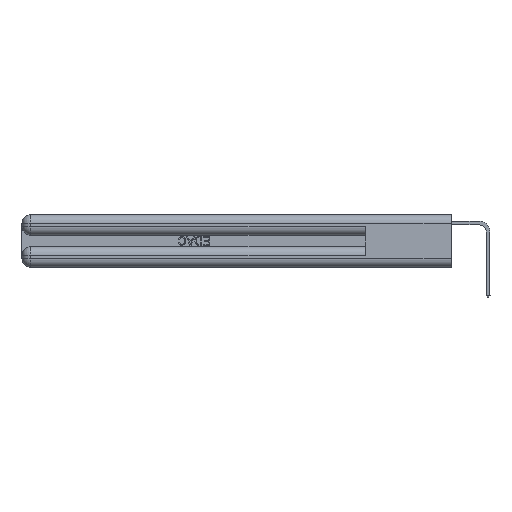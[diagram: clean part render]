
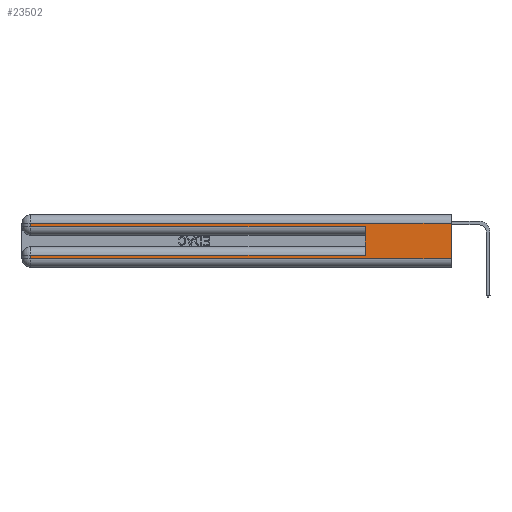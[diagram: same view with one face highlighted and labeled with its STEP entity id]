
A CAD part, left-side view. The second image highlights one B-rep face of the part: STEP entity #23502.
In plain terms, the highlighted planar face has unit normal (-1, 0, 0).
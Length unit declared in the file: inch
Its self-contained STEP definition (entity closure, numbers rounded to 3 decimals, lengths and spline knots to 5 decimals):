
#76 = VECTOR ( 'NONE', #25563, 39.37008 ) ;
#184 = CARTESIAN_POINT ( 'NONE',  ( 0., 2.94, 0.37 ) ) ;
#191 = VERTEX_POINT ( 'NONE', #11091 ) ;
#522 = CARTESIAN_POINT ( 'NONE',  ( 0., 0., 0.37 ) ) ;
#659 = ORIENTED_EDGE ( 'NONE', *, *, #31729, .T. ) ;
#1191 = CARTESIAN_POINT ( 'NONE',  ( 0., 2.94, 0.285 ) ) ;
#1357 = CARTESIAN_POINT ( 'NONE',  ( 0., 0.6, 0.285 ) ) ;
#1620 = ORIENTED_EDGE ( 'NONE', *, *, #3179, .T. ) ;
#1854 = ORIENTED_EDGE ( 'NONE', *, *, #27636, .F. ) ;
#2759 = LINE ( 'NONE', #522, #27994 ) ;
#3179 = EDGE_CURVE ( 'NONE', #11725, #24315, #15937, .T. ) ;
#3372 = VERTEX_POINT ( 'NONE', #1191 ) ;
#3619 = CARTESIAN_POINT ( 'NONE',  ( 0., 2.94, 0.085 ) ) ;
#3758 = EDGE_CURVE ( 'NONE', #26322, #11779, #14314, .T. ) ;
#4474 = EDGE_CURVE ( 'NONE', #24315, #31148, #29423, .T. ) ;
#5207 = EDGE_CURVE ( 'NONE', #33127, #3372, #30733, .T. ) ;
#6445 = VECTOR ( 'NONE', #21344, 39.37008 ) ;
#6697 = VECTOR ( 'NONE', #28147, 39.37008 ) ;
#7281 = DIRECTION ( 'NONE',  ( 1., 0., 0. ) ) ;
#8001 = ORIENTED_EDGE ( 'NONE', *, *, #3758, .F. ) ;
#8358 = VECTOR ( 'NONE', #28224, 39.37008 ) ;
#8670 = DIRECTION ( 'NONE',  ( 0., -1., 0. ) ) ;
#9128 = CARTESIAN_POINT ( 'NONE',  ( 0., 0.6, 0.145 ) ) ;
#9309 = EDGE_CURVE ( 'NONE', #3372, #11779, #12222, .T. ) ;
#9751 = ORIENTED_EDGE ( 'NONE', *, *, #4474, .T. ) ;
#11083 = CARTESIAN_POINT ( 'NONE',  ( 0., 0.6, 0.085 ) ) ;
#11091 = CARTESIAN_POINT ( 'NONE',  ( 0., 0., 0.31 ) ) ;
#11560 = CARTESIAN_POINT ( 'NONE',  ( 0., 2.94, 0.06 ) ) ;
#11604 = CARTESIAN_POINT ( 'NONE',  ( 0., 0., 0.06 ) ) ;
#11725 = VERTEX_POINT ( 'NONE', #3619 ) ;
#11779 = VERTEX_POINT ( 'NONE', #1357 ) ;
#11814 = CARTESIAN_POINT ( 'NONE',  ( 0., 0., 0.31 ) ) ;
#12222 = LINE ( 'NONE', #33140, #21683 ) ;
#12746 = CARTESIAN_POINT ( 'NONE',  ( 0., 0., 0.06 ) ) ;
#13017 = CARTESIAN_POINT ( 'NONE',  ( 0., 0., 0.37 ) ) ;
#13352 = DIRECTION ( 'NONE',  ( 0., 0., -1. ) ) ;
#14314 = LINE ( 'NONE', #9128, #6697 ) ;
#15551 = VECTOR ( 'NONE', #8670, 39.37008 ) ;
#15937 = LINE ( 'NONE', #184, #6445 ) ;
#17080 = DIRECTION ( 'NONE',  ( 0., -1., 0. ) ) ;
#17611 = CARTESIAN_POINT ( 'NONE',  ( 0., 2.94, 0.37 ) ) ;
#19448 = ORIENTED_EDGE ( 'NONE', *, *, #21286, .T. ) ;
#20329 = EDGE_LOOP ( 'NONE', ( #1854, #659, #26509, #27151, #8001, #19448, #1620, #9751 ) ) ;
#21286 = EDGE_CURVE ( 'NONE', #26322, #11725, #23200, .T. ) ;
#21344 = DIRECTION ( 'NONE',  ( 0., 0., -1. ) ) ;
#21683 = VECTOR ( 'NONE', #17080, 39.37008 ) ;
#23200 = LINE ( 'NONE', #33733, #31613 ) ;
#23502 = ADVANCED_FACE ( 'NONE', ( #28411 ), #31165, .F. ) ;
#23600 = DIRECTION ( 'NONE',  ( 0., 0., -1. ) ) ;
#24315 = VERTEX_POINT ( 'NONE', #11560 ) ;
#25563 = DIRECTION ( 'NONE',  ( 0., 0., -1. ) ) ;
#26322 = VERTEX_POINT ( 'NONE', #11083 ) ;
#26509 = ORIENTED_EDGE ( 'NONE', *, *, #5207, .T. ) ;
#27151 = ORIENTED_EDGE ( 'NONE', *, *, #9309, .T. ) ;
#27636 = EDGE_CURVE ( 'NONE', #191, #31148, #2759, .T. ) ;
#27994 = VECTOR ( 'NONE', #13352, 39.37008 ) ;
#28147 = DIRECTION ( 'NONE',  ( 0., 0., 1. ) ) ;
#28224 = DIRECTION ( 'NONE',  ( 0., 1., 0. ) ) ;
#28411 = FACE_OUTER_BOUND ( 'NONE', #20329, .T. ) ;
#28886 = DIRECTION ( 'NONE',  ( 0., 1., 0. ) ) ;
#29423 = LINE ( 'NONE', #11604, #15551 ) ;
#30733 = LINE ( 'NONE', #17611, #76 ) ;
#31148 = VERTEX_POINT ( 'NONE', #12746 ) ;
#31165 = PLANE ( 'NONE',  #31198 ) ;
#31198 = AXIS2_PLACEMENT_3D ( 'NONE', #13017, #7281, #23600 ) ;
#31274 = CARTESIAN_POINT ( 'NONE',  ( 0., 2.94, 0.31 ) ) ;
#31613 = VECTOR ( 'NONE', #28886, 39.37008 ) ;
#31729 = EDGE_CURVE ( 'NONE', #191, #33127, #33431, .T. ) ;
#33127 = VERTEX_POINT ( 'NONE', #31274 ) ;
#33140 = CARTESIAN_POINT ( 'NONE',  ( 0., 0., 0.285 ) ) ;
#33431 = LINE ( 'NONE', #11814, #8358 ) ;
#33733 = CARTESIAN_POINT ( 'NONE',  ( 0., 0., 0.085 ) ) ;
